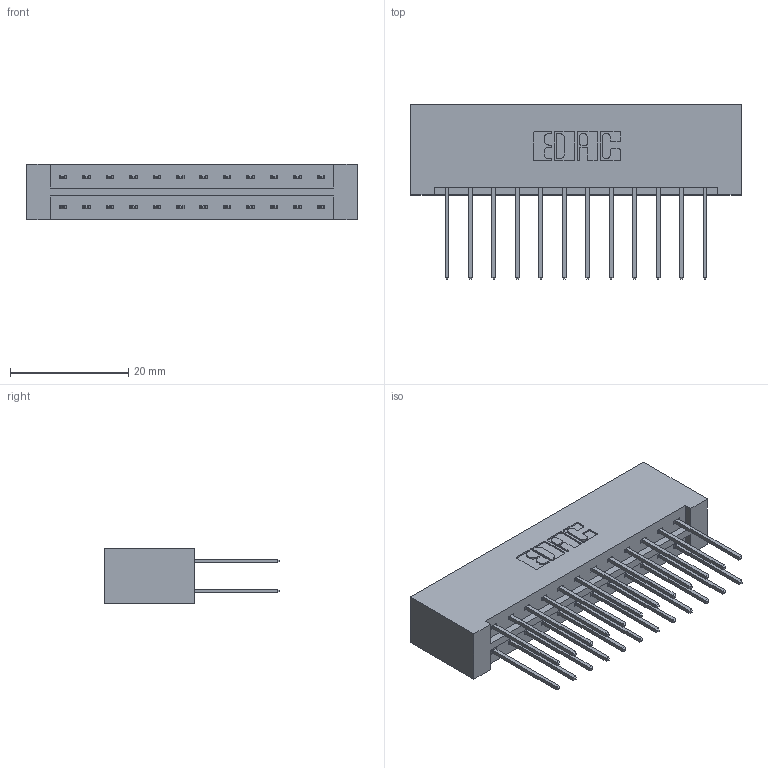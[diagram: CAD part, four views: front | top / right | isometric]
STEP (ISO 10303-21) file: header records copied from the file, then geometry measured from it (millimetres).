
FILE_DESCRIPTION (( 'STEP AP203' ), '1' );
FILE_NAME ('333-024-540-201.STEP', '2018-08-02T04:42:16', ( '' ), ( '' ), 'SwSTEP 2.0', 'SolidWorks 2016', '' );
FILE_SCHEMA (( 'CONFIG_CONTROL_DESIGN' ));
Length unit declared in the file: inch
Products named in the file (3): 333 Part_Lugless; 345-292-001_345-293-140; 333-024-540-201
Assembly tree (25 placements, depth 2):
  333-024-540-201
    333 Part_Lugless
    345-292-001_345-293-140  x24
Bounding box: 55.8 x 29.47 x 9.4 mm (x, y, z)
Volume: 6139.9 mm3; surface area: 7407.5 mm2
Topology: 25 solids, 25 shells, 1354 faces, 4007 edges, 2638 vertices
Faces by surface type: plane 930, cylinder 424
Entity records: 11341 total; most frequent: CARTESIAN_POINT 1914, ORIENTED_EDGE 1850, DIRECTION 1681, EDGE_CURVE 925, VECTOR 805, LINE 805, VERTEX_POINT 614, AXIS2_PLACEMENT_3D 438
